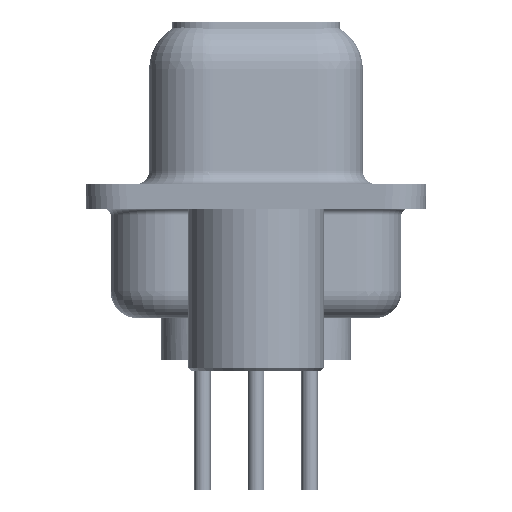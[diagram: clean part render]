
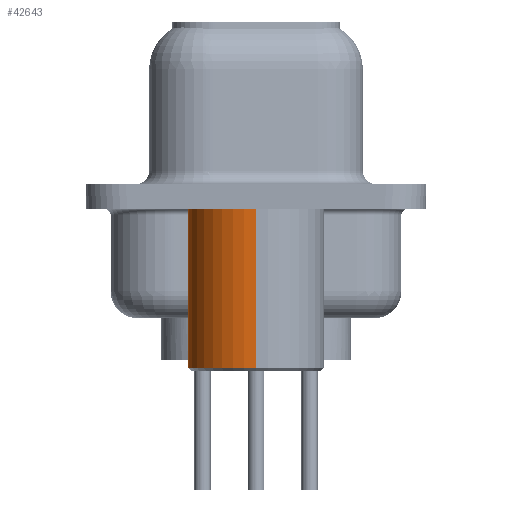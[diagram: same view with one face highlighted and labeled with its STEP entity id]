
A CAD part, left-side view. The second image highlights one B-rep face of the part: STEP entity #42643.
In plain terms, the highlighted cylindrical face has radius 2.5 mm (diameter 5 mm), a partial arc.
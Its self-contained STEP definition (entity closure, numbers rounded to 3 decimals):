
#989 = CARTESIAN_POINT ( 'NONE',  ( 0., 0., -0.45 ) ) ;
#3521 = VECTOR ( 'NONE', #46828, 1000. ) ;
#3854 = DIRECTION ( 'NONE',  ( 0., 0., 1. ) ) ;
#5005 = DIRECTION ( 'NONE',  ( 0., 0., 1. ) ) ;
#5390 = CARTESIAN_POINT ( 'NONE',  ( 2.5, 0., -6.35 ) ) ;
#5921 = DIRECTION ( 'NONE',  ( 0., 0., 1. ) ) ;
#6165 = CARTESIAN_POINT ( 'NONE',  ( 0., 0., 0.581 ) ) ;
#9106 = CARTESIAN_POINT ( 'NONE',  ( -2.5, 0., -6.35 ) ) ;
#9139 = AXIS2_PLACEMENT_3D ( 'NONE', #30458, #22744, #44722 ) ;
#10583 = CARTESIAN_POINT ( 'NONE',  ( -2.5, 0., 0.581 ) ) ;
#11640 = EDGE_CURVE ( 'NONE', #19255, #26103, #27644, .T. ) ;
#13497 = LINE ( 'NONE', #10583, #3521 ) ;
#13873 = EDGE_LOOP ( 'NONE', ( #32628, #36927, #20176, #41901 ) ) ;
#14645 = CIRCLE ( 'NONE', #32398, 2.5 ) ;
#19255 = VERTEX_POINT ( 'NONE', #5390 ) ;
#19730 = LINE ( 'NONE', #19978, #44223 ) ;
#19978 = CARTESIAN_POINT ( 'NONE',  ( 2.5, 0., 0.581 ) ) ;
#20176 = ORIENTED_EDGE ( 'NONE', *, *, #37550, .F. ) ;
#20634 = VERTEX_POINT ( 'NONE', #23104 ) ;
#22744 = DIRECTION ( 'NONE',  ( 0., 0., 1. ) ) ;
#23104 = CARTESIAN_POINT ( 'NONE',  ( -2.5, 0., -0.45 ) ) ;
#25043 = EDGE_CURVE ( 'NONE', #19255, #26935, #19730, .T. ) ;
#26103 = VERTEX_POINT ( 'NONE', #9106 ) ;
#26876 = EDGE_CURVE ( 'NONE', #26103, #20634, #13497, .T. ) ;
#26935 = VERTEX_POINT ( 'NONE', #36637 ) ;
#27644 = CIRCLE ( 'NONE', #9139, 2.5 ) ;
#30458 = CARTESIAN_POINT ( 'NONE',  ( 0., 0., -6.35 ) ) ;
#32398 = AXIS2_PLACEMENT_3D ( 'NONE', #989, #3854, #37632 ) ;
#32628 = ORIENTED_EDGE ( 'NONE', *, *, #11640, .T. ) ;
#34648 = CYLINDRICAL_SURFACE ( 'NONE', #39734, 2.5 ) ;
#35610 = DIRECTION ( 'NONE',  ( 1., 0., 0. ) ) ;
#36637 = CARTESIAN_POINT ( 'NONE',  ( 2.5, 0., -0.45 ) ) ;
#36927 = ORIENTED_EDGE ( 'NONE', *, *, #26876, .T. ) ;
#37550 = EDGE_CURVE ( 'NONE', #26935, #20634, #14645, .T. ) ;
#37632 = DIRECTION ( 'NONE',  ( 1., 0., 0. ) ) ;
#39734 = AXIS2_PLACEMENT_3D ( 'NONE', #6165, #5921, #35610 ) ;
#41901 = ORIENTED_EDGE ( 'NONE', *, *, #25043, .F. ) ;
#42383 = FACE_OUTER_BOUND ( 'NONE', #13873, .T. ) ;
#42643 = ADVANCED_FACE ( 'NONE', ( #42383 ), #34648, .T. ) ;
#44223 = VECTOR ( 'NONE', #5005, 1000. ) ;
#44722 = DIRECTION ( 'NONE',  ( 1., 0., 0. ) ) ;
#46828 = DIRECTION ( 'NONE',  ( 0., 0., 1. ) ) ;
